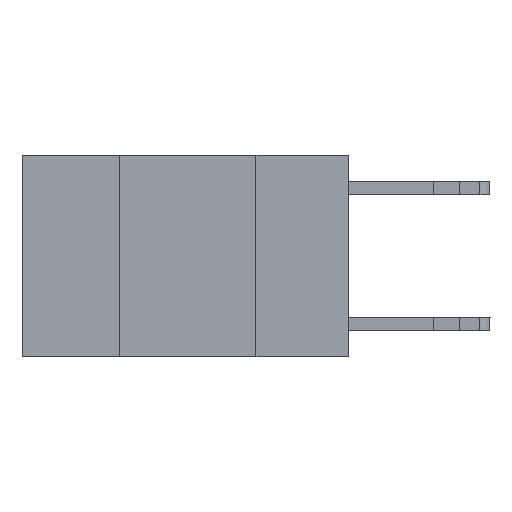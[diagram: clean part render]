
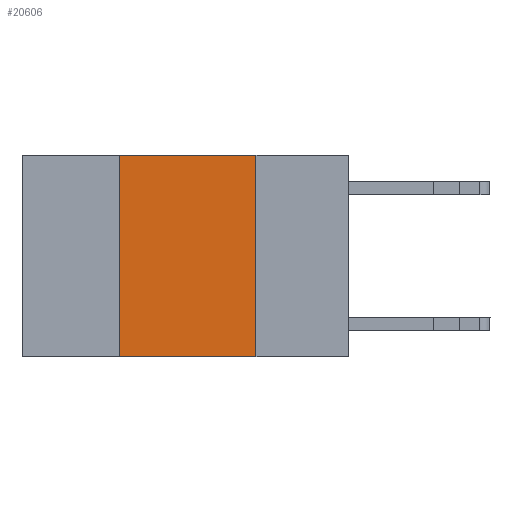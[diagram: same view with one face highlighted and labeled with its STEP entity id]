
A CAD part, left-side view. The second image highlights one B-rep face of the part: STEP entity #20606.
In plain terms, the highlighted planar face has unit normal (-1, 0, 0).
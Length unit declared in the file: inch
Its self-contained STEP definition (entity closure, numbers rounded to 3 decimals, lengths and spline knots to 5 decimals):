
#1086 = EDGE_CURVE ( 'NONE', #8228, #8490, #16287, .T. ) ;
#1338 = EDGE_CURVE ( 'NONE', #8228, #13332, #13798, .T. ) ;
#1599 = FACE_OUTER_BOUND ( 'NONE', #18666, .T. ) ;
#1782 = DIRECTION ( 'NONE',  ( 0., 0., -1. ) ) ;
#3689 = CARTESIAN_POINT ( 'NONE',  ( 0., 0.42, 0. ) ) ;
#3853 = CARTESIAN_POINT ( 'NONE',  ( 0., 0.42, -0.37 ) ) ;
#3947 = EDGE_CURVE ( 'NONE', #17612, #8490, #15304, .T. ) ;
#4532 = ORIENTED_EDGE ( 'NONE', *, *, #1086, .T. ) ;
#4758 = CARTESIAN_POINT ( 'NONE',  ( 0., 0.17, 0. ) ) ;
#5105 = DIRECTION ( 'NONE',  ( 0., 0., 1. ) ) ;
#6020 = ORIENTED_EDGE ( 'NONE', *, *, #9479, .F. ) ;
#7439 = PLANE ( 'NONE',  #22439 ) ;
#8228 = VERTEX_POINT ( 'NONE', #3853 ) ;
#8490 = VERTEX_POINT ( 'NONE', #23098 ) ;
#8809 = VECTOR ( 'NONE', #22648, 39.37008 ) ;
#9131 = LINE ( 'NONE', #23125, #8809 ) ;
#9189 = ORIENTED_EDGE ( 'NONE', *, *, #1338, .F. ) ;
#9479 = EDGE_CURVE ( 'NONE', #13332, #17612, #9131, .T. ) ;
#10504 = CARTESIAN_POINT ( 'NONE',  ( 0., 0.42, 0. ) ) ;
#10538 = ORIENTED_EDGE ( 'NONE', *, *, #3947, .F. ) ;
#10844 = CARTESIAN_POINT ( 'NONE',  ( 0., 0.6, -0.37 ) ) ;
#12771 = DIRECTION ( 'NONE',  ( 1., 0., 0. ) ) ;
#13263 = DIRECTION ( 'NONE',  ( 0., -1., 0. ) ) ;
#13332 = VERTEX_POINT ( 'NONE', #3689 ) ;
#13744 = VECTOR ( 'NONE', #5105, 39.37008 ) ;
#13798 = LINE ( 'NONE', #10504, #13744 ) ;
#15249 = VECTOR ( 'NONE', #22202, 39.37008 ) ;
#15304 = LINE ( 'NONE', #19238, #15249 ) ;
#16287 = LINE ( 'NONE', #10844, #16395 ) ;
#16395 = VECTOR ( 'NONE', #13263, 39.37008 ) ;
#17612 = VERTEX_POINT ( 'NONE', #4758 ) ;
#18666 = EDGE_LOOP ( 'NONE', ( #10538, #6020, #9189, #4532 ) ) ;
#19238 = CARTESIAN_POINT ( 'NONE',  ( 0., 0.17, 0. ) ) ;
#20606 = ADVANCED_FACE ( 'NONE', ( #1599 ), #7439, .F. ) ;
#22202 = DIRECTION ( 'NONE',  ( 0., 0., -1. ) ) ;
#22439 = AXIS2_PLACEMENT_3D ( 'NONE', #23097, #12771, #1782 ) ;
#22648 = DIRECTION ( 'NONE',  ( 0., -1., 0. ) ) ;
#23097 = CARTESIAN_POINT ( 'NONE',  ( 0., 0.6, 0. ) ) ;
#23098 = CARTESIAN_POINT ( 'NONE',  ( 0., 0.17, -0.37 ) ) ;
#23125 = CARTESIAN_POINT ( 'NONE',  ( 0., 0.6, 0. ) ) ;
